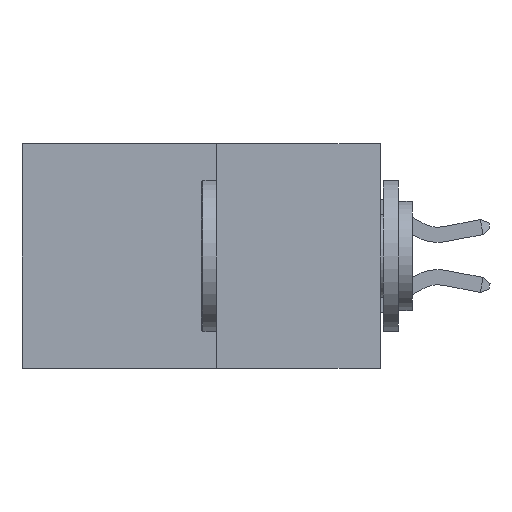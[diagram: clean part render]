
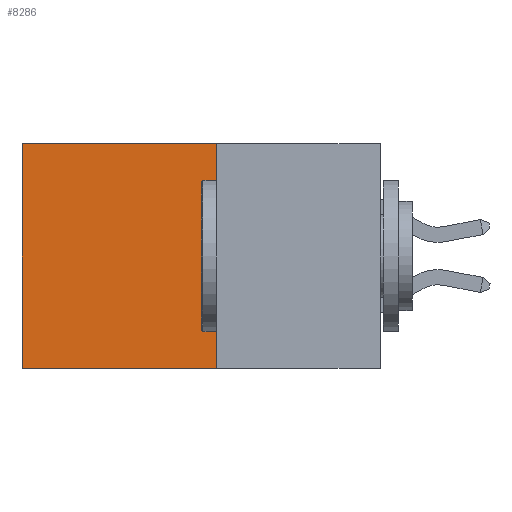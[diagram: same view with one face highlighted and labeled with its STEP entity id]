
A CAD part, left-side view. The second image highlights one B-rep face of the part: STEP entity #8286.
In plain terms, the highlighted planar face has unit normal (-1, 0, 0).
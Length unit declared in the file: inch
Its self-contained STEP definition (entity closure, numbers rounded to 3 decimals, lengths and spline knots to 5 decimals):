
#487 = DIRECTION ( 'NONE',  ( 1., 0., 0. ) ) ;
#697 = DIRECTION ( 'NONE',  ( 0., 0., -1. ) ) ;
#3170 = ORIENTED_EDGE ( 'NONE', *, *, #12712, .F. ) ;
#4639 = DIRECTION ( 'NONE',  ( 0., 0., -1. ) ) ;
#5215 = CARTESIAN_POINT ( 'NONE',  ( 0.277, 0.27, -0.37 ) ) ;
#7828 = FACE_OUTER_BOUND ( 'NONE', #10332, .T. ) ;
#7938 = VECTOR ( 'NONE', #697, 39.37008 ) ;
#8286 = ADVANCED_FACE ( 'NONE', ( #7828 ), #14429, .F. ) ;
#9778 = VECTOR ( 'NONE', #4639, 39.37008 ) ;
#9914 = LINE ( 'NONE', #23766, #21425 ) ;
#10332 = EDGE_LOOP ( 'NONE', ( #16620, #3170, #27061, #15772 ) ) ;
#10726 = CARTESIAN_POINT ( 'NONE',  ( 0.277, 0.27, 0. ) ) ;
#11731 = VERTEX_POINT ( 'NONE', #29809 ) ;
#12712 = EDGE_CURVE ( 'NONE', #18854, #25236, #9914, .T. ) ;
#14004 = LINE ( 'NONE', #28272, #7938 ) ;
#14429 = PLANE ( 'NONE',  #23877 ) ;
#15772 = ORIENTED_EDGE ( 'NONE', *, *, #25233, .T. ) ;
#16620 = ORIENTED_EDGE ( 'NONE', *, *, #20300, .T. ) ;
#16801 = DIRECTION ( 'NONE',  ( 0., 0., -1. ) ) ;
#16814 = CARTESIAN_POINT ( 'NONE',  ( 0.277, 0.27, -0.37 ) ) ;
#17411 = LINE ( 'NONE', #29193, #18107 ) ;
#17905 = CARTESIAN_POINT ( 'NONE',  ( 0.277, 0.59, -0.37 ) ) ;
#18107 = VECTOR ( 'NONE', #24608, 39.37008 ) ;
#18854 = VERTEX_POINT ( 'NONE', #16814 ) ;
#19147 = DIRECTION ( 'NONE',  ( 0., 1., 0. ) ) ;
#19797 = VERTEX_POINT ( 'NONE', #10726 ) ;
#20300 = EDGE_CURVE ( 'NONE', #11731, #25236, #14004, .T. ) ;
#20692 = CARTESIAN_POINT ( 'NONE',  ( 0.277, 0.27, -0.37 ) ) ;
#21274 = LINE ( 'NONE', #20692, #9778 ) ;
#21425 = VECTOR ( 'NONE', #19147, 39.37008 ) ;
#23766 = CARTESIAN_POINT ( 'NONE',  ( 0.277, 0.27, -0.37 ) ) ;
#23877 = AXIS2_PLACEMENT_3D ( 'NONE', #5215, #487, #16801 ) ;
#24608 = DIRECTION ( 'NONE',  ( 0., 1., 0. ) ) ;
#25233 = EDGE_CURVE ( 'NONE', #19797, #11731, #17411, .T. ) ;
#25236 = VERTEX_POINT ( 'NONE', #17905 ) ;
#26451 = EDGE_CURVE ( 'NONE', #19797, #18854, #21274, .T. ) ;
#27061 = ORIENTED_EDGE ( 'NONE', *, *, #26451, .F. ) ;
#28272 = CARTESIAN_POINT ( 'NONE',  ( 0.277, 0.59, -0.37 ) ) ;
#29193 = CARTESIAN_POINT ( 'NONE',  ( 0.277, 0.27, 0. ) ) ;
#29809 = CARTESIAN_POINT ( 'NONE',  ( 0.277, 0.59, 0. ) ) ;
